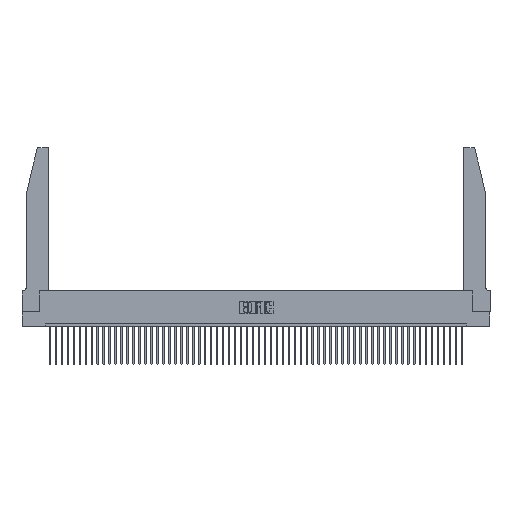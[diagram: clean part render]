
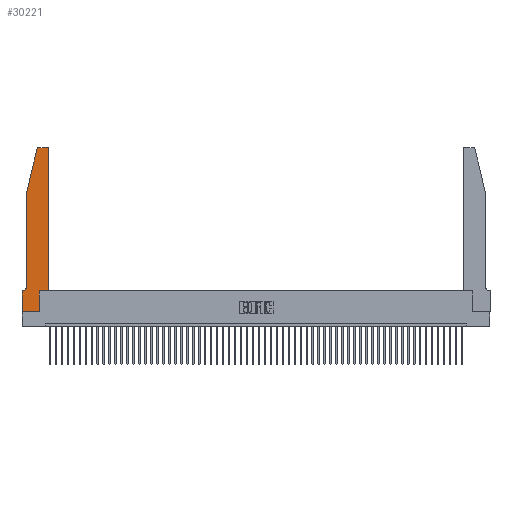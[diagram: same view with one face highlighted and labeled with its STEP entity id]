
A CAD part, top view. The second image highlights one B-rep face of the part: STEP entity #30221.
In plain terms, the highlighted planar face has unit normal (0, 0, 1).
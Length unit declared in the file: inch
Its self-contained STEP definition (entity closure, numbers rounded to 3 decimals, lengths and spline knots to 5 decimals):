
#334 = VERTEX_POINT ( 'NONE', #17429 ) ;
#738 = ORIENTED_EDGE ( 'NONE', *, *, #26145, .T. ) ;
#928 = DIRECTION ( 'NONE',  ( 1., 0., 0. ) ) ;
#1184 = VECTOR ( 'NONE', #5783, 39.37008 ) ;
#1489 = EDGE_CURVE ( 'NONE', #26146, #17412, #11532, .T. ) ;
#2403 = ORIENTED_EDGE ( 'NONE', *, *, #5686, .T. ) ;
#2502 = CARTESIAN_POINT ( 'NONE',  ( 0.4505, 0.35, 0.37 ) ) ;
#3497 = VERTEX_POINT ( 'NONE', #7562 ) ;
#3807 = CARTESIAN_POINT ( 'NONE',  ( 0.4205, 2.72, 0.37 ) ) ;
#4151 = CIRCLE ( 'NONE', #51226, 0.07 ) ;
#4587 = LINE ( 'NONE', #51462, #1184 ) ;
#4705 = LINE ( 'NONE', #16250, #35951 ) ;
#5686 = EDGE_CURVE ( 'NONE', #25392, #12066, #4705, .T. ) ;
#5783 = DIRECTION ( 'NONE',  ( 1., 0., 0. ) ) ;
#5954 = VECTOR ( 'NONE', #43896, 39.37008 ) ;
#6013 = PLANE ( 'NONE',  #46160 ) ;
#6089 = CARTESIAN_POINT ( 'NONE',  ( 0.0755, 0.42, 0.37 ) ) ;
#6253 = CARTESIAN_POINT ( 'NONE',  ( 0.0055, 0.42, 0.37 ) ) ;
#6336 = EDGE_CURVE ( 'NONE', #15914, #25392, #25985, .T. ) ;
#6504 = ORIENTED_EDGE ( 'NONE', *, *, #48272, .T. ) ;
#7562 = CARTESIAN_POINT ( 'NONE',  ( 0.284, 2.75, 0.37 ) ) ;
#7842 = CARTESIAN_POINT ( 'NONE',  ( 0., 0., 0.37 ) ) ;
#7923 = EDGE_CURVE ( 'NONE', #33742, #334, #33663, .T. ) ;
#8234 = ORIENTED_EDGE ( 'NONE', *, *, #23703, .T. ) ;
#8598 = VECTOR ( 'NONE', #44810, 39.37008 ) ;
#9578 = CIRCLE ( 'NONE', #46010, 0.03 ) ;
#11193 = VECTOR ( 'NONE', #52060, 39.37008 ) ;
#11532 = LINE ( 'NONE', #44110, #36189 ) ;
#12066 = VERTEX_POINT ( 'NONE', #39764 ) ;
#12101 = ORIENTED_EDGE ( 'NONE', *, *, #1489, .T. ) ;
#12111 = CARTESIAN_POINT ( 'NONE',  ( 0.25487, 2.72718, 0.37 ) ) ;
#12308 = DIRECTION ( 'NONE',  ( 0., 0., 1. ) ) ;
#12350 = LINE ( 'NONE', #49848, #19470 ) ;
#12579 = EDGE_CURVE ( 'NONE', #26787, #15914, #39064, .T. ) ;
#12685 = DIRECTION ( 'NONE',  ( 0., -1., 0. ) ) ;
#12974 = DIRECTION ( 'NONE',  ( 1., 0., 0. ) ) ;
#14389 = DIRECTION ( 'NONE',  ( 0., 0., 1. ) ) ;
#15059 = VECTOR ( 'NONE', #12974, 39.37008 ) ;
#15914 = VERTEX_POINT ( 'NONE', #49505 ) ;
#16250 = CARTESIAN_POINT ( 'NONE',  ( 0.4505, 0.35, 0.37 ) ) ;
#16821 = VECTOR ( 'NONE', #12685, 39.37008 ) ;
#17041 = CARTESIAN_POINT ( 'NONE',  ( 0.4205, 2.75, 0.37 ) ) ;
#17412 = VERTEX_POINT ( 'NONE', #6089 ) ;
#17429 = CARTESIAN_POINT ( 'NONE',  ( 0., 0., 0.37 ) ) ;
#17524 = DIRECTION ( 'NONE',  ( -1., 0., 0. ) ) ;
#18534 = DIRECTION ( 'NONE',  ( 1., 0., 0. ) ) ;
#19470 = VECTOR ( 'NONE', #17524, 39.37008 ) ;
#19650 = CARTESIAN_POINT ( 'NONE',  ( 0.0755, 2., 0.37 ) ) ;
#19873 = DIRECTION ( 'NONE',  ( 0., -1., 0. ) ) ;
#22936 = EDGE_LOOP ( 'NONE', ( #738, #46184, #51912, #12101, #24897, #24304, #25933, #8234, #24328, #52546, #2403, #6504 ) ) ;
#22990 = EDGE_CURVE ( 'NONE', #41781, #26146, #46676, .T. ) ;
#23703 = EDGE_CURVE ( 'NONE', #334, #26787, #4587, .T. ) ;
#24304 = ORIENTED_EDGE ( 'NONE', *, *, #47207, .T. ) ;
#24328 = ORIENTED_EDGE ( 'NONE', *, *, #12579, .T. ) ;
#24897 = ORIENTED_EDGE ( 'NONE', *, *, #38013, .T. ) ;
#25010 = CARTESIAN_POINT ( 'NONE',  ( 0.284, 2.72, 0.37 ) ) ;
#25392 = VERTEX_POINT ( 'NONE', #43397 ) ;
#25933 = ORIENTED_EDGE ( 'NONE', *, *, #7923, .T. ) ;
#25985 = LINE ( 'NONE', #2502, #15059 ) ;
#26145 = EDGE_CURVE ( 'NONE', #36331, #3497, #35886, .T. ) ;
#26146 = VERTEX_POINT ( 'NONE', #19650 ) ;
#26787 = VERTEX_POINT ( 'NONE', #42807 ) ;
#27121 = DIRECTION ( 'NONE',  ( -1., 0., 0. ) ) ;
#28477 = AXIS2_PLACEMENT_3D ( 'NONE', #25010, #46431, #928 ) ;
#30221 = ADVANCED_FACE ( 'NONE', ( #52893 ), #6013, .T. ) ;
#32092 = CIRCLE ( 'NONE', #28477, 0.03 ) ;
#33663 = LINE ( 'NONE', #7842, #16821 ) ;
#33742 = VERTEX_POINT ( 'NONE', #44612 ) ;
#34604 = CARTESIAN_POINT ( 'NONE',  ( 0.0055, 0.35, 0.37 ) ) ;
#35293 = DIRECTION ( 'NONE',  ( 0., 0., -1. ) ) ;
#35886 = LINE ( 'NONE', #49281, #8598 ) ;
#35951 = VECTOR ( 'NONE', #49370, 39.37008 ) ;
#36189 = VECTOR ( 'NONE', #19873, 39.37008 ) ;
#36331 = VERTEX_POINT ( 'NONE', #17041 ) ;
#37153 = EDGE_CURVE ( 'NONE', #3497, #41781, #32092, .T. ) ;
#38013 = EDGE_CURVE ( 'NONE', #17412, #49161, #4151, .T. ) ;
#39064 = LINE ( 'NONE', #44264, #5954 ) ;
#39221 = CARTESIAN_POINT ( 'NONE',  ( 0., 0.35, 0.37 ) ) ;
#39764 = CARTESIAN_POINT ( 'NONE',  ( 0.4505, 2.72, 0.37 ) ) ;
#41144 = DIRECTION ( 'NONE',  ( 1., 0., 0. ) ) ;
#41781 = VERTEX_POINT ( 'NONE', #12111 ) ;
#42807 = CARTESIAN_POINT ( 'NONE',  ( 0.2865, 0., 0.37 ) ) ;
#43397 = CARTESIAN_POINT ( 'NONE',  ( 0.4505, 0.35, 0.37 ) ) ;
#43896 = DIRECTION ( 'NONE',  ( 0., 1., 0. ) ) ;
#44110 = CARTESIAN_POINT ( 'NONE',  ( 0.0755, 2., 0.37 ) ) ;
#44264 = CARTESIAN_POINT ( 'NONE',  ( 0.2865, 0.35, 0.37 ) ) ;
#44612 = CARTESIAN_POINT ( 'NONE',  ( 0., 0.35, 0.37 ) ) ;
#44810 = DIRECTION ( 'NONE',  ( -1., 0., 0. ) ) ;
#46010 = AXIS2_PLACEMENT_3D ( 'NONE', #3807, #12308, #41144 ) ;
#46160 = AXIS2_PLACEMENT_3D ( 'NONE', #39221, #14389, #18534 ) ;
#46184 = ORIENTED_EDGE ( 'NONE', *, *, #37153, .T. ) ;
#46431 = DIRECTION ( 'NONE',  ( 0., 0., 1. ) ) ;
#46676 = LINE ( 'NONE', #47247, #11193 ) ;
#47207 = EDGE_CURVE ( 'NONE', #49161, #33742, #12350, .T. ) ;
#47247 = CARTESIAN_POINT ( 'NONE',  ( 0.0755, 2., 0.37 ) ) ;
#48272 = EDGE_CURVE ( 'NONE', #12066, #36331, #9578, .T. ) ;
#49161 = VERTEX_POINT ( 'NONE', #34604 ) ;
#49281 = CARTESIAN_POINT ( 'NONE',  ( 0.2605, 2.75, 0.37 ) ) ;
#49370 = DIRECTION ( 'NONE',  ( 0., 1., 0. ) ) ;
#49505 = CARTESIAN_POINT ( 'NONE',  ( 0.2865, 0.35, 0.37 ) ) ;
#49848 = CARTESIAN_POINT ( 'NONE',  ( 0.0755, 0.35, 0.37 ) ) ;
#51226 = AXIS2_PLACEMENT_3D ( 'NONE', #6253, #35293, #27121 ) ;
#51462 = CARTESIAN_POINT ( 'NONE',  ( 0., 0., 0.37 ) ) ;
#51912 = ORIENTED_EDGE ( 'NONE', *, *, #22990, .T. ) ;
#52060 = DIRECTION ( 'NONE',  ( -0.239, -0.971, 0. ) ) ;
#52546 = ORIENTED_EDGE ( 'NONE', *, *, #6336, .T. ) ;
#52893 = FACE_OUTER_BOUND ( 'NONE', #22936, .T. ) ;
